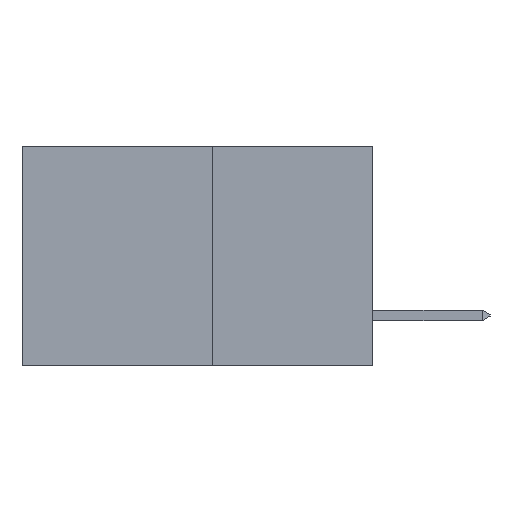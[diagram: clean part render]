
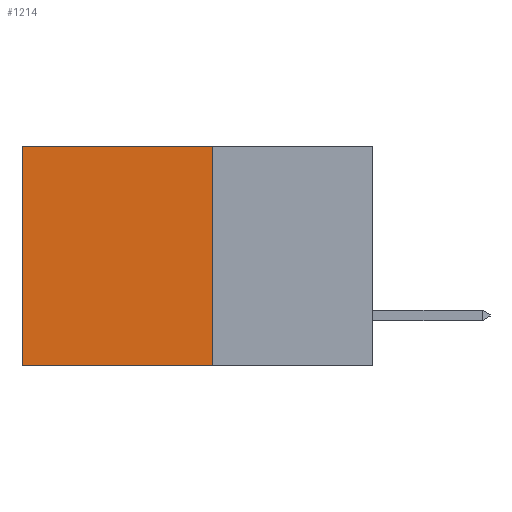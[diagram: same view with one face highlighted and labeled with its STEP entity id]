
A CAD part, left-side view. The second image highlights one B-rep face of the part: STEP entity #1214.
In plain terms, the highlighted planar face has unit normal (-1, 0, 0).
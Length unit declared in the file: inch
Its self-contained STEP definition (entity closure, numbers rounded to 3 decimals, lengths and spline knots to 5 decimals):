
#175 = VECTOR ( 'NONE', #10451, 39.37008 ) ;
#264 = DIRECTION ( 'NONE',  ( 0., 0., -1. ) ) ;
#875 = LINE ( 'NONE', #5914, #6531 ) ;
#1214 = ADVANCED_FACE ( 'NONE', ( #3643 ), #10029, .F. ) ;
#1217 = EDGE_CURVE ( 'NONE', #13249, #8098, #875, .T. ) ;
#2315 = CARTESIAN_POINT ( 'NONE',  ( 0.277, 0.27, -0.37 ) ) ;
#2938 = LINE ( 'NONE', #3177, #175 ) ;
#3000 = EDGE_CURVE ( 'NONE', #9909, #13249, #8978, .T. ) ;
#3019 = EDGE_CURVE ( 'NONE', #9909, #3473, #2938, .T. ) ;
#3177 = CARTESIAN_POINT ( 'NONE',  ( 0.277, 0.27, 0. ) ) ;
#3473 = VERTEX_POINT ( 'NONE', #8706 ) ;
#3643 = FACE_OUTER_BOUND ( 'NONE', #11797, .T. ) ;
#3892 = LINE ( 'NONE', #9812, #6791 ) ;
#5897 = CARTESIAN_POINT ( 'NONE',  ( 0.277, 0.59, -0.37 ) ) ;
#5914 = CARTESIAN_POINT ( 'NONE',  ( 0.277, 0.27, -0.37 ) ) ;
#6531 = VECTOR ( 'NONE', #8182, 39.37008 ) ;
#6791 = VECTOR ( 'NONE', #264, 39.37008 ) ;
#6804 = ORIENTED_EDGE ( 'NONE', *, *, #1217, .F. ) ;
#7490 = ORIENTED_EDGE ( 'NONE', *, *, #3000, .F. ) ;
#7831 = ORIENTED_EDGE ( 'NONE', *, *, #3019, .T. ) ;
#8098 = VERTEX_POINT ( 'NONE', #5897 ) ;
#8182 = DIRECTION ( 'NONE',  ( 0., 1., 0. ) ) ;
#8706 = CARTESIAN_POINT ( 'NONE',  ( 0.277, 0.59, 0. ) ) ;
#8777 = DIRECTION ( 'NONE',  ( 0., 0., -1. ) ) ;
#8978 = LINE ( 'NONE', #2315, #11746 ) ;
#9566 = EDGE_CURVE ( 'NONE', #3473, #8098, #3892, .T. ) ;
#9602 = ORIENTED_EDGE ( 'NONE', *, *, #9566, .T. ) ;
#9812 = CARTESIAN_POINT ( 'NONE',  ( 0.277, 0.59, -0.37 ) ) ;
#9909 = VERTEX_POINT ( 'NONE', #10337 ) ;
#10029 = PLANE ( 'NONE',  #12215 ) ;
#10082 = DIRECTION ( 'NONE',  ( 1., 0., 0. ) ) ;
#10167 = CARTESIAN_POINT ( 'NONE',  ( 0.277, 0.27, -0.37 ) ) ;
#10337 = CARTESIAN_POINT ( 'NONE',  ( 0.277, 0.27, 0. ) ) ;
#10451 = DIRECTION ( 'NONE',  ( 0., 1., 0. ) ) ;
#11407 = DIRECTION ( 'NONE',  ( 0., 0., -1. ) ) ;
#11746 = VECTOR ( 'NONE', #8777, 39.37008 ) ;
#11797 = EDGE_LOOP ( 'NONE', ( #9602, #6804, #7490, #7831 ) ) ;
#12215 = AXIS2_PLACEMENT_3D ( 'NONE', #10167, #10082, #11407 ) ;
#13249 = VERTEX_POINT ( 'NONE', #13536 ) ;
#13536 = CARTESIAN_POINT ( 'NONE',  ( 0.277, 0.27, -0.37 ) ) ;
